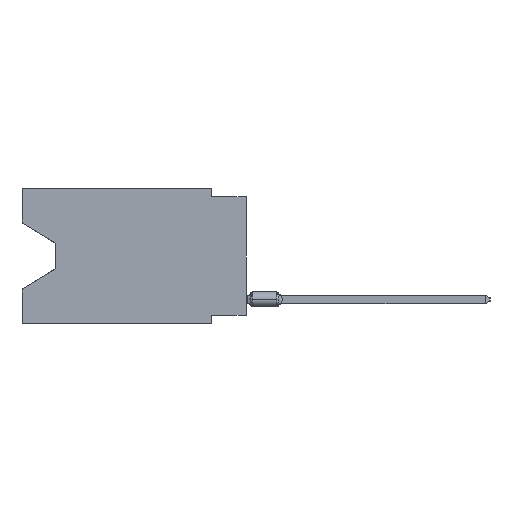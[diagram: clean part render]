
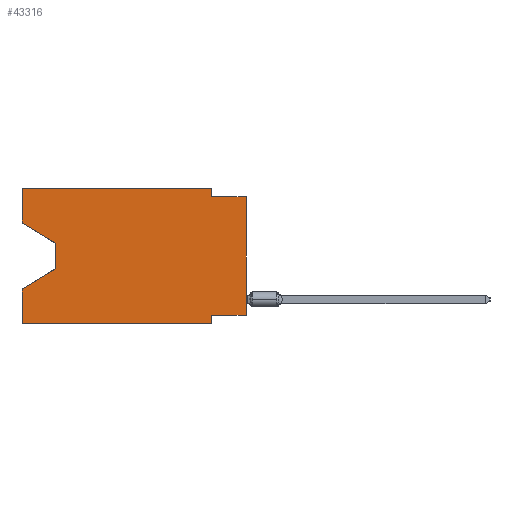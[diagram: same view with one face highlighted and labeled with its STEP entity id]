
A CAD part, left-side view. The second image highlights one B-rep face of the part: STEP entity #43316.
In plain terms, the highlighted planar face has unit normal (-1, 0, 0).
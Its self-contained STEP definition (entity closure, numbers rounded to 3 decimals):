
#1949 = PLANE ( 'NONE',  #71458 ) ;
#3007 = EDGE_CURVE ( 'NONE', #48788, #33200, #69277, .T. ) ;
#3928 = ORIENTED_EDGE ( 'NONE', *, *, #10663, .F. ) ;
#6074 = CARTESIAN_POINT ( 'NONE',  ( 0., 2.54, -0.635 ) ) ;
#6134 = VECTOR ( 'NONE', #26205, 1000. ) ;
#6724 = EDGE_CURVE ( 'NONE', #33297, #77992, #6727, .T. ) ;
#6727 = LINE ( 'NONE', #30982, #56008 ) ;
#7422 = CARTESIAN_POINT ( 'NONE',  ( 0., 16.383, -7.36 ) ) ;
#7623 = DIRECTION ( 'NONE',  ( 0., -1., 0. ) ) ;
#10349 = CARTESIAN_POINT ( 'NONE',  ( 0., 2.54, 0. ) ) ;
#10663 = EDGE_CURVE ( 'NONE', #68173, #73731, #12890, .T. ) ;
#11688 = DIRECTION ( 'NONE',  ( 0., 0., 1. ) ) ;
#11850 = CARTESIAN_POINT ( 'NONE',  ( 0., 13.97, -4.013 ) ) ;
#12558 = DIRECTION ( 'NONE',  ( 0., -0.855, -0.519 ) ) ;
#12870 = ORIENTED_EDGE ( 'NONE', *, *, #14187, .F. ) ;
#12890 = LINE ( 'NONE', #19148, #18641 ) ;
#13241 = CARTESIAN_POINT ( 'NONE',  ( 0., 0., -0.635 ) ) ;
#14187 = EDGE_CURVE ( 'NONE', #44933, #15469, #33941, .T. ) ;
#14263 = EDGE_CURVE ( 'NONE', #77992, #48788, #47298, .T. ) ;
#15469 = VERTEX_POINT ( 'NONE', #79939 ) ;
#15711 = DIRECTION ( 'NONE',  ( 0., 0., 1. ) ) ;
#16513 = CARTESIAN_POINT ( 'NONE',  ( 0., 16.383, 0. ) ) ;
#16937 = DIRECTION ( 'NONE',  ( 0., 0., -1. ) ) ;
#18476 = CARTESIAN_POINT ( 'NONE',  ( 0., 2.54, 0. ) ) ;
#18641 = VECTOR ( 'NONE', #70162, 1000. ) ;
#19062 = VECTOR ( 'NONE', #15711, 1000. ) ;
#19148 = CARTESIAN_POINT ( 'NONE',  ( 0., 16.383, 0. ) ) ;
#20779 = DIRECTION ( 'NONE',  ( 1., 0., 0. ) ) ;
#21421 = CARTESIAN_POINT ( 'NONE',  ( 0., 16.383, -9.906 ) ) ;
#21648 = VECTOR ( 'NONE', #53585, 1000. ) ;
#22332 = ORIENTED_EDGE ( 'NONE', *, *, #71004, .F. ) ;
#22659 = LINE ( 'NONE', #34764, #21648 ) ;
#24026 = LINE ( 'NONE', #50314, #79044 ) ;
#24326 = ORIENTED_EDGE ( 'NONE', *, *, #71566, .F. ) ;
#24356 = CARTESIAN_POINT ( 'NONE',  ( 0., 2.54, -9.906 ) ) ;
#25802 = VERTEX_POINT ( 'NONE', #6074 ) ;
#26205 = DIRECTION ( 'NONE',  ( 0., 0.855, -0.519 ) ) ;
#27475 = VERTEX_POINT ( 'NONE', #68599 ) ;
#29597 = CARTESIAN_POINT ( 'NONE',  ( 0., 0., -9.271 ) ) ;
#30117 = ORIENTED_EDGE ( 'NONE', *, *, #14263, .T. ) ;
#30982 = CARTESIAN_POINT ( 'NONE',  ( 0., 16.383, -2.546 ) ) ;
#31026 = EDGE_CURVE ( 'NONE', #27475, #33200, #22659, .T. ) ;
#32542 = CARTESIAN_POINT ( 'NONE',  ( 0., 16.383, 0. ) ) ;
#33200 = VERTEX_POINT ( 'NONE', #7422 ) ;
#33297 = VERTEX_POINT ( 'NONE', #45044 ) ;
#33941 = LINE ( 'NONE', #78285, #53033 ) ;
#34764 = CARTESIAN_POINT ( 'NONE',  ( 0., 16.383, 0. ) ) ;
#34994 = LINE ( 'NONE', #10349, #65796 ) ;
#36968 = EDGE_CURVE ( 'NONE', #25802, #55247, #56393, .T. ) ;
#37509 = ORIENTED_EDGE ( 'NONE', *, *, #57327, .T. ) ;
#37534 = DIRECTION ( 'NONE',  ( 0., -1., 0. ) ) ;
#38333 = VECTOR ( 'NONE', #37534, 1000. ) ;
#39550 = CARTESIAN_POINT ( 'NONE',  ( 0., 16.383, 0. ) ) ;
#40197 = CARTESIAN_POINT ( 'NONE',  ( 0., 13.97, -4.013 ) ) ;
#41532 = ORIENTED_EDGE ( 'NONE', *, *, #36968, .F. ) ;
#41648 = EDGE_CURVE ( 'NONE', #44933, #55247, #43440, .T. ) ;
#42512 = ORIENTED_EDGE ( 'NONE', *, *, #72035, .F. ) ;
#43316 = ADVANCED_FACE ( 'NONE', ( #70941 ), #1949, .F. ) ;
#43440 = LINE ( 'NONE', #68970, #64519 ) ;
#43989 = LINE ( 'NONE', #21421, #58344 ) ;
#44933 = VERTEX_POINT ( 'NONE', #29597 ) ;
#45044 = CARTESIAN_POINT ( 'NONE',  ( 0., 16.383, -2.546 ) ) ;
#47298 = LINE ( 'NONE', #40197, #48890 ) ;
#47555 = DIRECTION ( 'NONE',  ( 0., 0., -1. ) ) ;
#48671 = LINE ( 'NONE', #16513, #19062 ) ;
#48788 = VERTEX_POINT ( 'NONE', #52386 ) ;
#48890 = VECTOR ( 'NONE', #54428, 1000. ) ;
#50314 = CARTESIAN_POINT ( 'NONE',  ( 0., 2.54, -9.906 ) ) ;
#52321 = ORIENTED_EDGE ( 'NONE', *, *, #31026, .F. ) ;
#52386 = CARTESIAN_POINT ( 'NONE',  ( 0., 13.97, -5.893 ) ) ;
#53033 = VECTOR ( 'NONE', #73255, 1000. ) ;
#53585 = DIRECTION ( 'NONE',  ( 0., 0., 1. ) ) ;
#54119 = VERTEX_POINT ( 'NONE', #24356 ) ;
#54428 = DIRECTION ( 'NONE',  ( 0., 0., -1. ) ) ;
#54512 = ORIENTED_EDGE ( 'NONE', *, *, #41648, .T. ) ;
#55247 = VERTEX_POINT ( 'NONE', #13241 ) ;
#56008 = VECTOR ( 'NONE', #12558, 1000. ) ;
#56393 = LINE ( 'NONE', #69345, #38333 ) ;
#56719 = CARTESIAN_POINT ( 'NONE',  ( 0., 13.97, -5.893 ) ) ;
#57327 = EDGE_CURVE ( 'NONE', #27475, #54119, #43989, .T. ) ;
#57562 = DIRECTION ( 'NONE',  ( 0., 0., -1. ) ) ;
#58344 = VECTOR ( 'NONE', #7623, 1000. ) ;
#61214 = EDGE_LOOP ( 'NONE', ( #82395, #30117, #76669, #52321, #37509, #22332, #12870, #54512, #41532, #24326, #3928, #42512 ) ) ;
#64519 = VECTOR ( 'NONE', #11688, 1000. ) ;
#65796 = VECTOR ( 'NONE', #47555, 1000. ) ;
#68173 = VERTEX_POINT ( 'NONE', #32542 ) ;
#68599 = CARTESIAN_POINT ( 'NONE',  ( 0., 16.383, -9.906 ) ) ;
#68970 = CARTESIAN_POINT ( 'NONE',  ( 0., 0., 0. ) ) ;
#69277 = LINE ( 'NONE', #56719, #6134 ) ;
#69345 = CARTESIAN_POINT ( 'NONE',  ( 0., 0., -0.635 ) ) ;
#70162 = DIRECTION ( 'NONE',  ( 0., -1., 0. ) ) ;
#70941 = FACE_OUTER_BOUND ( 'NONE', #61214, .T. ) ;
#71004 = EDGE_CURVE ( 'NONE', #15469, #54119, #24026, .T. ) ;
#71458 = AXIS2_PLACEMENT_3D ( 'NONE', #39550, #20779, #57562 ) ;
#71566 = EDGE_CURVE ( 'NONE', #73731, #25802, #34994, .T. ) ;
#72035 = EDGE_CURVE ( 'NONE', #33297, #68173, #48671, .T. ) ;
#73255 = DIRECTION ( 'NONE',  ( 0., 1., 0. ) ) ;
#73731 = VERTEX_POINT ( 'NONE', #18476 ) ;
#76669 = ORIENTED_EDGE ( 'NONE', *, *, #3007, .T. ) ;
#77992 = VERTEX_POINT ( 'NONE', #11850 ) ;
#78285 = CARTESIAN_POINT ( 'NONE',  ( 0., 0., -9.271 ) ) ;
#79044 = VECTOR ( 'NONE', #16937, 1000. ) ;
#79939 = CARTESIAN_POINT ( 'NONE',  ( 0., 2.54, -9.271 ) ) ;
#82395 = ORIENTED_EDGE ( 'NONE', *, *, #6724, .T. ) ;
